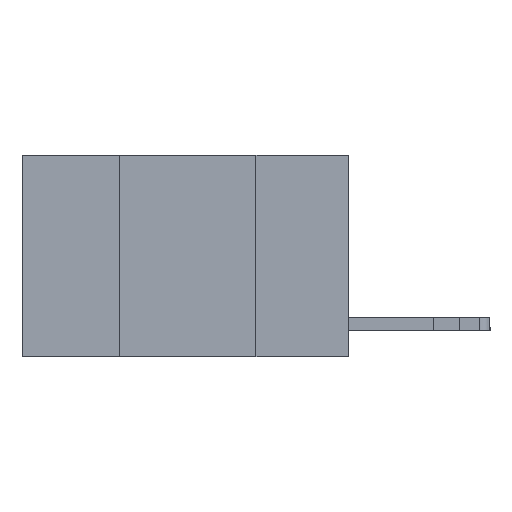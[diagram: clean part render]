
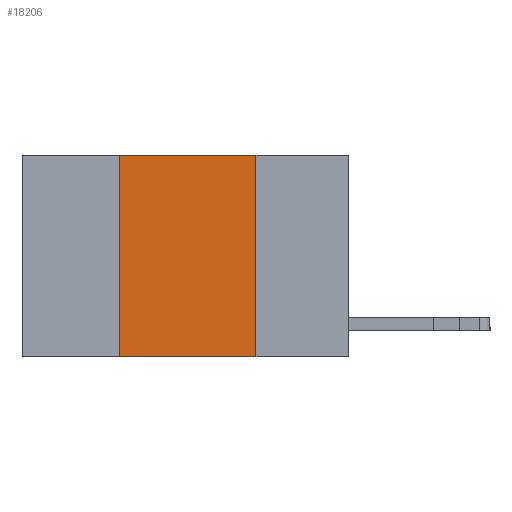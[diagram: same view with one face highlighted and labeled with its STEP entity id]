
A CAD part, left-side view. The second image highlights one B-rep face of the part: STEP entity #18206.
In plain terms, the highlighted planar face has unit normal (-1, 0, 0).
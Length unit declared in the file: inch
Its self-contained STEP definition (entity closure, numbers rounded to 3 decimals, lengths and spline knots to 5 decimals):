
#275 = PLANE ( 'NONE',  #4528 ) ;
#1087 = EDGE_CURVE ( 'NONE', #11121, #9220, #12610, .T. ) ;
#1908 = VECTOR ( 'NONE', #17666, 39.37008 ) ;
#1962 = CARTESIAN_POINT ( 'NONE',  ( 0., 0.42, 0. ) ) ;
#2443 = CARTESIAN_POINT ( 'NONE',  ( 0., 0.6, 0. ) ) ;
#2488 = CARTESIAN_POINT ( 'NONE',  ( 0., 0.42, 0. ) ) ;
#3130 = EDGE_CURVE ( 'NONE', #12556, #9220, #12069, .T. ) ;
#3634 = CARTESIAN_POINT ( 'NONE',  ( 0., 0.17, 0. ) ) ;
#3637 = VECTOR ( 'NONE', #12707, 39.37008 ) ;
#4528 = AXIS2_PLACEMENT_3D ( 'NONE', #6228, #6021, #4821 ) ;
#4565 = DIRECTION ( 'NONE',  ( 0., -1., 0. ) ) ;
#4737 = CARTESIAN_POINT ( 'NONE',  ( 0., 0.17, -0.37 ) ) ;
#4821 = DIRECTION ( 'NONE',  ( 0., 0., -1. ) ) ;
#5136 = ORIENTED_EDGE ( 'NONE', *, *, #9936, .F. ) ;
#5347 = EDGE_CURVE ( 'NONE', #12556, #18358, #17624, .T. ) ;
#6021 = DIRECTION ( 'NONE',  ( 1., 0., 0. ) ) ;
#6228 = CARTESIAN_POINT ( 'NONE',  ( 0., 0.6, 0. ) ) ;
#6477 = ORIENTED_EDGE ( 'NONE', *, *, #5347, .F. ) ;
#6928 = DIRECTION ( 'NONE',  ( 0., 0., 1. ) ) ;
#9220 = VERTEX_POINT ( 'NONE', #4737 ) ;
#9936 = EDGE_CURVE ( 'NONE', #18358, #11121, #10046, .T. ) ;
#10046 = LINE ( 'NONE', #2443, #1908 ) ;
#11121 = VERTEX_POINT ( 'NONE', #3634 ) ;
#12069 = LINE ( 'NONE', #18112, #13992 ) ;
#12276 = EDGE_LOOP ( 'NONE', ( #18175, #5136, #6477, #16893 ) ) ;
#12449 = VECTOR ( 'NONE', #6928, 39.37008 ) ;
#12517 = CARTESIAN_POINT ( 'NONE',  ( 0., 0.17, 0. ) ) ;
#12556 = VERTEX_POINT ( 'NONE', #12861 ) ;
#12610 = LINE ( 'NONE', #12517, #3637 ) ;
#12707 = DIRECTION ( 'NONE',  ( 0., 0., -1. ) ) ;
#12861 = CARTESIAN_POINT ( 'NONE',  ( 0., 0.42, -0.37 ) ) ;
#13845 = FACE_OUTER_BOUND ( 'NONE', #12276, .T. ) ;
#13992 = VECTOR ( 'NONE', #4565, 39.37008 ) ;
#16893 = ORIENTED_EDGE ( 'NONE', *, *, #3130, .T. ) ;
#17624 = LINE ( 'NONE', #2488, #12449 ) ;
#17666 = DIRECTION ( 'NONE',  ( 0., -1., 0. ) ) ;
#18112 = CARTESIAN_POINT ( 'NONE',  ( 0., 0.6, -0.37 ) ) ;
#18175 = ORIENTED_EDGE ( 'NONE', *, *, #1087, .F. ) ;
#18206 = ADVANCED_FACE ( 'NONE', ( #13845 ), #275, .F. ) ;
#18358 = VERTEX_POINT ( 'NONE', #1962 ) ;
